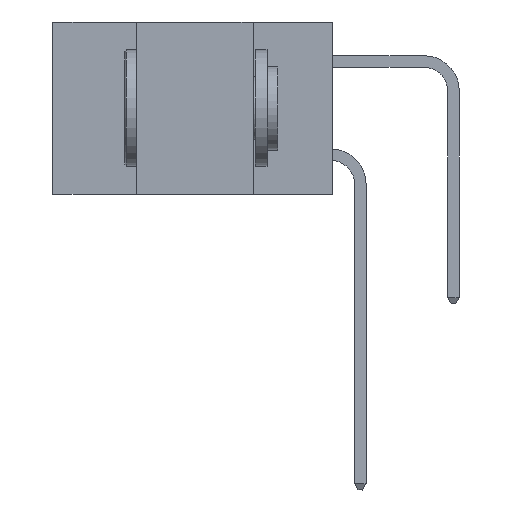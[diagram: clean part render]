
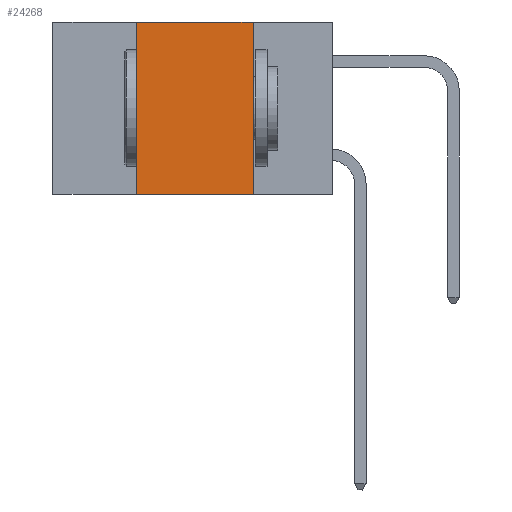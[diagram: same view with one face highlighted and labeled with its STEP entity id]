
A CAD part, left-side view. The second image highlights one B-rep face of the part: STEP entity #24268.
In plain terms, the highlighted planar face has unit normal (-1, 0, 0).
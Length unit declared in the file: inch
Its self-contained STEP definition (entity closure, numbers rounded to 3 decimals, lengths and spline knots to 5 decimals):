
#680 = CARTESIAN_POINT ( 'NONE',  ( 0., 0.42, 0. ) ) ;
#2507 = ORIENTED_EDGE ( 'NONE', *, *, #3612, .T. ) ;
#3612 = EDGE_CURVE ( 'NONE', #17763, #16709, #9658, .T. ) ;
#3901 = VECTOR ( 'NONE', #18752, 39.37008 ) ;
#6063 = CARTESIAN_POINT ( 'NONE',  ( 0., 0.6, 0. ) ) ;
#6576 = LINE ( 'NONE', #18553, #22577 ) ;
#7706 = DIRECTION ( 'NONE',  ( 0., -1., 0. ) ) ;
#9658 = LINE ( 'NONE', #24546, #3901 ) ;
#9707 = CARTESIAN_POINT ( 'NONE',  ( 0., 0.17, 0. ) ) ;
#10861 = EDGE_CURVE ( 'NONE', #17763, #19608, #23466, .T. ) ;
#12363 = VECTOR ( 'NONE', #27047, 39.37008 ) ;
#12474 = FACE_OUTER_BOUND ( 'NONE', #27574, .T. ) ;
#12586 = VECTOR ( 'NONE', #15905, 39.37008 ) ;
#12624 = DIRECTION ( 'NONE',  ( 0., 0., -1. ) ) ;
#15905 = DIRECTION ( 'NONE',  ( 0., 0., 1. ) ) ;
#16184 = AXIS2_PLACEMENT_3D ( 'NONE', #6063, #25624, #12624 ) ;
#16709 = VERTEX_POINT ( 'NONE', #18354 ) ;
#16718 = EDGE_CURVE ( 'NONE', #22524, #16709, #18139, .T. ) ;
#16752 = EDGE_CURVE ( 'NONE', #19608, #22524, #6576, .T. ) ;
#17763 = VERTEX_POINT ( 'NONE', #24479 ) ;
#18139 = LINE ( 'NONE', #9707, #12363 ) ;
#18354 = CARTESIAN_POINT ( 'NONE',  ( 0., 0.17, -0.37 ) ) ;
#18553 = CARTESIAN_POINT ( 'NONE',  ( 0., 0.6, 0. ) ) ;
#18752 = DIRECTION ( 'NONE',  ( 0., -1., 0. ) ) ;
#19608 = VERTEX_POINT ( 'NONE', #19615 ) ;
#19615 = CARTESIAN_POINT ( 'NONE',  ( 0., 0.42, 0. ) ) ;
#21262 = PLANE ( 'NONE',  #16184 ) ;
#22524 = VERTEX_POINT ( 'NONE', #23911 ) ;
#22577 = VECTOR ( 'NONE', #7706, 39.37008 ) ;
#23466 = LINE ( 'NONE', #680, #12586 ) ;
#23911 = CARTESIAN_POINT ( 'NONE',  ( 0., 0.17, 0. ) ) ;
#24268 = ADVANCED_FACE ( 'NONE', ( #12474 ), #21262, .F. ) ;
#24479 = CARTESIAN_POINT ( 'NONE',  ( 0., 0.42, -0.37 ) ) ;
#24546 = CARTESIAN_POINT ( 'NONE',  ( 0., 0.6, -0.37 ) ) ;
#24555 = ORIENTED_EDGE ( 'NONE', *, *, #16752, .F. ) ;
#24889 = ORIENTED_EDGE ( 'NONE', *, *, #16718, .F. ) ;
#25624 = DIRECTION ( 'NONE',  ( 1., 0., 0. ) ) ;
#25914 = ORIENTED_EDGE ( 'NONE', *, *, #10861, .F. ) ;
#27047 = DIRECTION ( 'NONE',  ( 0., 0., -1. ) ) ;
#27574 = EDGE_LOOP ( 'NONE', ( #24889, #24555, #25914, #2507 ) ) ;
